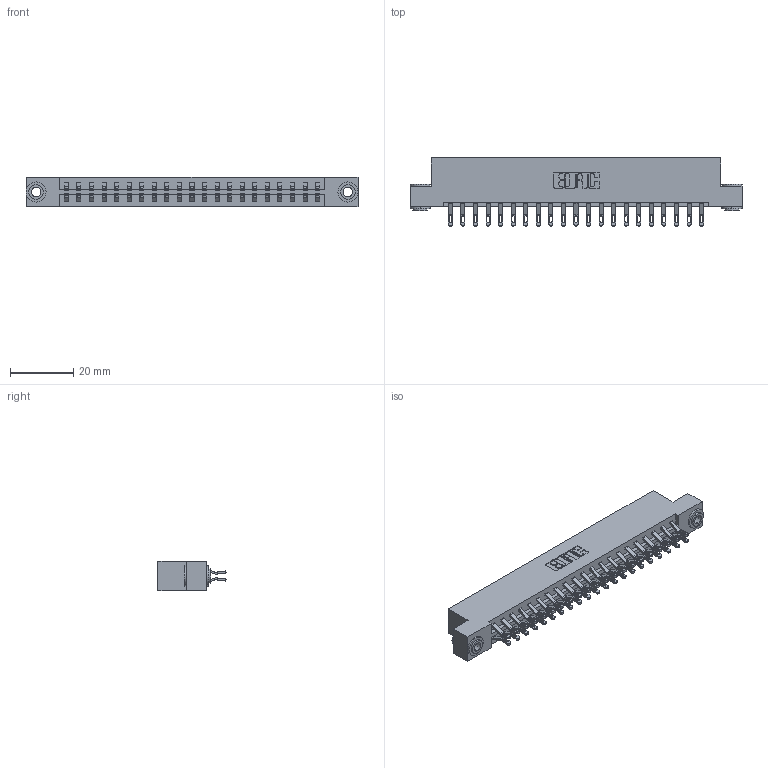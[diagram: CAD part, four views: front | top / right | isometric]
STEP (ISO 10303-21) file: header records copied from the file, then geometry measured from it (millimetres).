
FILE_DESCRIPTION (( 'STEP AP203' ), '1' );
FILE_NAME ('833-042-555-203.STEP', '2020-06-03T22:11:31', ( '' ), ( '' ), 'SwSTEP 2.0', 'SolidWorks 2020', '' );
FILE_SCHEMA (( 'CONFIG_CONTROL_DESIGN' ));
Length unit declared in the file: inch
Products named in the file (4): 345-250-002_345-250-002-102; 833 Part_Flush - .156 Dia - TH; 345-292-001_555 Tail; 833-042-555-203
Assembly tree (45 placements, depth 2):
  833-042-555-203
    833 Part_Flush - .156 Dia - TH
    345-292-001_555 Tail  x42
    345-250-002_345-250-002-102  x2
Bounding box: 104.75 x 21.47 x 9.4 mm (x, y, z)
Volume: 10639.2 mm3; surface area: 13029 mm2
Topology: 45 solids, 45 shells, 2588 faces, 8073 edges, 5378 vertices
Faces by surface type: plane 1508, cylinder 1072, cone 8
Entity records: 17202 total; most frequent: CARTESIAN_POINT 2887, ORIENTED_EDGE 2786, DIRECTION 2507, EDGE_CURVE 1393, VECTOR 1221, LINE 1221, VERTEX_POINT 926, AXIS2_PLACEMENT_3D 643
